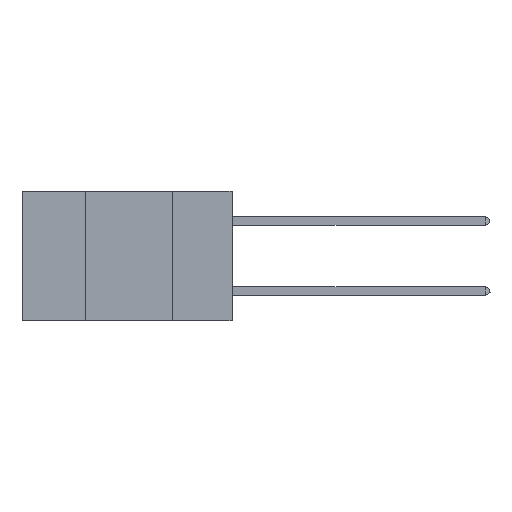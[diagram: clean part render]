
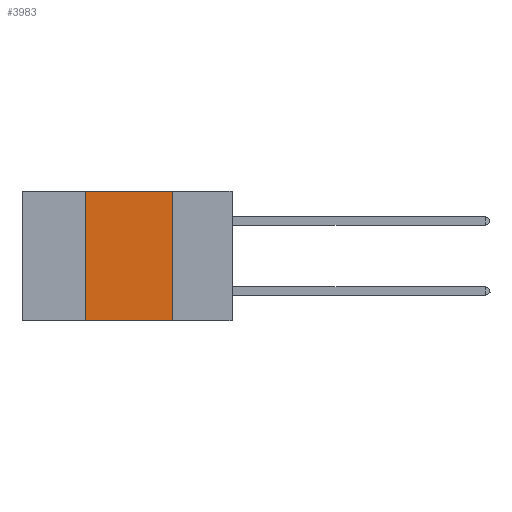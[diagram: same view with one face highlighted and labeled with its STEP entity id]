
A CAD part, left-side view. The second image highlights one B-rep face of the part: STEP entity #3983.
In plain terms, the highlighted planar face has unit normal (-1, 0, 0).
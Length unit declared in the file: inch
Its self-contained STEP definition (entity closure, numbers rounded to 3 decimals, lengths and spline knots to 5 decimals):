
#834 = LINE ( 'NONE', #21954, #10452 ) ;
#1013 = CARTESIAN_POINT ( 'NONE',  ( 0., 0.17, 0. ) ) ;
#1803 = VERTEX_POINT ( 'NONE', #24432 ) ;
#2398 = DIRECTION ( 'NONE',  ( 0., 0., -1. ) ) ;
#3983 = ADVANCED_FACE ( 'NONE', ( #7595 ), #32372, .F. ) ;
#7595 = FACE_OUTER_BOUND ( 'NONE', #16902, .T. ) ;
#8384 = ORIENTED_EDGE ( 'NONE', *, *, #20464, .T. ) ;
#8896 = ORIENTED_EDGE ( 'NONE', *, *, #31049, .F. ) ;
#8978 = DIRECTION ( 'NONE',  ( 0., -1., 0. ) ) ;
#10452 = VECTOR ( 'NONE', #19186, 39.37008 ) ;
#11441 = AXIS2_PLACEMENT_3D ( 'NONE', #15065, #15324, #18246 ) ;
#11585 = DIRECTION ( 'NONE',  ( 0., -1., 0. ) ) ;
#12317 = EDGE_CURVE ( 'NONE', #1803, #30797, #834, .T. ) ;
#15065 = CARTESIAN_POINT ( 'NONE',  ( 0., 0.6, 0. ) ) ;
#15082 = VERTEX_POINT ( 'NONE', #33507 ) ;
#15324 = DIRECTION ( 'NONE',  ( 1., 0., 0. ) ) ;
#15915 = CARTESIAN_POINT ( 'NONE',  ( 0., 0.42, 0. ) ) ;
#16902 = EDGE_LOOP ( 'NONE', ( #8896, #30079, #24418, #8384 ) ) ;
#18246 = DIRECTION ( 'NONE',  ( 0., 0., -1. ) ) ;
#18790 = LINE ( 'NONE', #26082, #20569 ) ;
#19186 = DIRECTION ( 'NONE',  ( 0., 0., 1. ) ) ;
#20464 = EDGE_CURVE ( 'NONE', #1803, #15082, #35082, .T. ) ;
#20569 = VECTOR ( 'NONE', #8978, 39.37008 ) ;
#21133 = CARTESIAN_POINT ( 'NONE',  ( 0., 0.17, 0. ) ) ;
#21954 = CARTESIAN_POINT ( 'NONE',  ( 0., 0.42, 0. ) ) ;
#22068 = EDGE_CURVE ( 'NONE', #30797, #22730, #18790, .T. ) ;
#22730 = VERTEX_POINT ( 'NONE', #21133 ) ;
#24418 = ORIENTED_EDGE ( 'NONE', *, *, #12317, .F. ) ;
#24432 = CARTESIAN_POINT ( 'NONE',  ( 0., 0.42, -0.37 ) ) ;
#26082 = CARTESIAN_POINT ( 'NONE',  ( 0., 0.6, 0. ) ) ;
#29687 = VECTOR ( 'NONE', #11585, 39.37008 ) ;
#30079 = ORIENTED_EDGE ( 'NONE', *, *, #22068, .F. ) ;
#30797 = VERTEX_POINT ( 'NONE', #15915 ) ;
#31049 = EDGE_CURVE ( 'NONE', #22730, #15082, #32666, .T. ) ;
#32372 = PLANE ( 'NONE',  #11441 ) ;
#32666 = LINE ( 'NONE', #1013, #34924 ) ;
#33507 = CARTESIAN_POINT ( 'NONE',  ( 0., 0.17, -0.37 ) ) ;
#34924 = VECTOR ( 'NONE', #2398, 39.37008 ) ;
#35082 = LINE ( 'NONE', #36335, #29687 ) ;
#36335 = CARTESIAN_POINT ( 'NONE',  ( 0., 0.6, -0.37 ) ) ;
